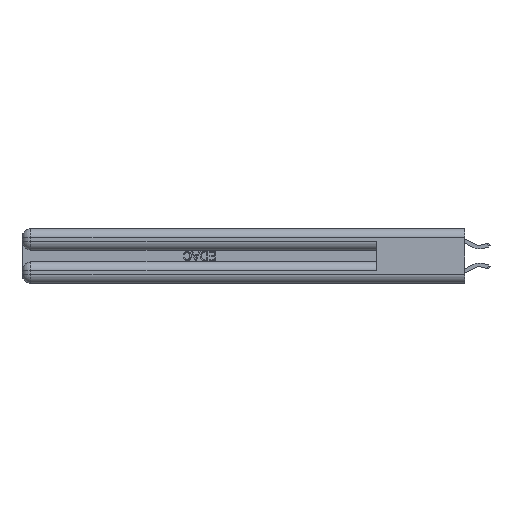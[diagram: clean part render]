
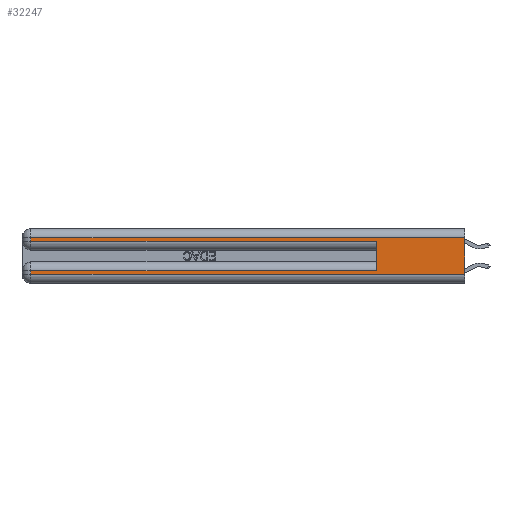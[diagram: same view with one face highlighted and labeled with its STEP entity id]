
A CAD part, left-side view. The second image highlights one B-rep face of the part: STEP entity #32247.
In plain terms, the highlighted planar face has unit normal (-1, 0, 0).
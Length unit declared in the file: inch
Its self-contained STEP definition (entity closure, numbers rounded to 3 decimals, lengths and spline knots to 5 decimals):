
#521 = VERTEX_POINT ( 'NONE', #4528 ) ;
#645 = CARTESIAN_POINT ( 'NONE',  ( 0., 0.6, 0.085 ) ) ;
#839 = CARTESIAN_POINT ( 'NONE',  ( 0., 0., 0.285 ) ) ;
#1564 = DIRECTION ( 'NONE',  ( 0., -1., 0. ) ) ;
#1755 = LINE ( 'NONE', #20086, #27776 ) ;
#1814 = AXIS2_PLACEMENT_3D ( 'NONE', #4807, #31588, #29104 ) ;
#2146 = CARTESIAN_POINT ( 'NONE',  ( 0., 2.94, 0.37 ) ) ;
#2331 = LINE ( 'NONE', #15736, #18131 ) ;
#2772 = LINE ( 'NONE', #21984, #14631 ) ;
#3386 = ORIENTED_EDGE ( 'NONE', *, *, #16109, .T. ) ;
#3832 = CARTESIAN_POINT ( 'NONE',  ( 0., 0., 0.31 ) ) ;
#3846 = VERTEX_POINT ( 'NONE', #17870 ) ;
#4039 = ORIENTED_EDGE ( 'NONE', *, *, #29134, .F. ) ;
#4528 = CARTESIAN_POINT ( 'NONE',  ( 0., 2.94, 0.06 ) ) ;
#4693 = EDGE_CURVE ( 'NONE', #20149, #20709, #12934, .T. ) ;
#4807 = CARTESIAN_POINT ( 'NONE',  ( 0., 0., 0.37 ) ) ;
#5538 = EDGE_CURVE ( 'NONE', #20709, #32707, #14271, .T. ) ;
#5596 = EDGE_CURVE ( 'NONE', #21968, #20149, #15321, .T. ) ;
#6369 = VECTOR ( 'NONE', #26561, 39.37008 ) ;
#7666 = ORIENTED_EDGE ( 'NONE', *, *, #15448, .F. ) ;
#8062 = CARTESIAN_POINT ( 'NONE',  ( 0., 0., 0.31 ) ) ;
#9660 = EDGE_LOOP ( 'NONE', ( #7666, #19116, #23951, #28795, #4039, #12200, #33163, #3386 ) ) ;
#11644 = DIRECTION ( 'NONE',  ( 0., -1., 0. ) ) ;
#12200 = ORIENTED_EDGE ( 'NONE', *, *, #12401, .T. ) ;
#12401 = EDGE_CURVE ( 'NONE', #13423, #26680, #2331, .T. ) ;
#12593 = CARTESIAN_POINT ( 'NONE',  ( 0., 2.94, 0.085 ) ) ;
#12934 = LINE ( 'NONE', #2146, #33450 ) ;
#13423 = VERTEX_POINT ( 'NONE', #645 ) ;
#13480 = LINE ( 'NONE', #21568, #13785 ) ;
#13690 = EDGE_CURVE ( 'NONE', #26680, #521, #31986, .T. ) ;
#13785 = VECTOR ( 'NONE', #31953, 39.37008 ) ;
#14271 = LINE ( 'NONE', #839, #33241 ) ;
#14631 = VECTOR ( 'NONE', #30089, 39.37008 ) ;
#15321 = LINE ( 'NONE', #3832, #25917 ) ;
#15400 = PLANE ( 'NONE',  #1814 ) ;
#15448 = EDGE_CURVE ( 'NONE', #21968, #3846, #13480, .T. ) ;
#15736 = CARTESIAN_POINT ( 'NONE',  ( 0., 0., 0.085 ) ) ;
#15806 = CARTESIAN_POINT ( 'NONE',  ( 0., 2.94, 0.37 ) ) ;
#16109 = EDGE_CURVE ( 'NONE', #521, #3846, #1755, .T. ) ;
#17154 = CARTESIAN_POINT ( 'NONE',  ( 0., 2.94, 0.31 ) ) ;
#17870 = CARTESIAN_POINT ( 'NONE',  ( 0., 0., 0.06 ) ) ;
#18131 = VECTOR ( 'NONE', #26308, 39.37008 ) ;
#19116 = ORIENTED_EDGE ( 'NONE', *, *, #5596, .T. ) ;
#20086 = CARTESIAN_POINT ( 'NONE',  ( 0., 0., 0.06 ) ) ;
#20149 = VERTEX_POINT ( 'NONE', #17154 ) ;
#20709 = VERTEX_POINT ( 'NONE', #34025 ) ;
#21568 = CARTESIAN_POINT ( 'NONE',  ( 0., 0., 0.37 ) ) ;
#21968 = VERTEX_POINT ( 'NONE', #8062 ) ;
#21984 = CARTESIAN_POINT ( 'NONE',  ( 0., 0.6, 0.145 ) ) ;
#23951 = ORIENTED_EDGE ( 'NONE', *, *, #4693, .T. ) ;
#25917 = VECTOR ( 'NONE', #28339, 39.37008 ) ;
#26308 = DIRECTION ( 'NONE',  ( 0., 1., 0. ) ) ;
#26561 = DIRECTION ( 'NONE',  ( 0., 0., -1. ) ) ;
#26680 = VERTEX_POINT ( 'NONE', #12593 ) ;
#27776 = VECTOR ( 'NONE', #1564, 39.37008 ) ;
#28339 = DIRECTION ( 'NONE',  ( 0., 1., 0. ) ) ;
#28795 = ORIENTED_EDGE ( 'NONE', *, *, #5538, .T. ) ;
#29104 = DIRECTION ( 'NONE',  ( 0., 0., -1. ) ) ;
#29134 = EDGE_CURVE ( 'NONE', #13423, #32707, #2772, .T. ) ;
#29243 = CARTESIAN_POINT ( 'NONE',  ( 0., 0.6, 0.285 ) ) ;
#30089 = DIRECTION ( 'NONE',  ( 0., 0., 1. ) ) ;
#31080 = DIRECTION ( 'NONE',  ( 0., 0., -1. ) ) ;
#31588 = DIRECTION ( 'NONE',  ( 1., 0., 0. ) ) ;
#31953 = DIRECTION ( 'NONE',  ( 0., 0., -1. ) ) ;
#31986 = LINE ( 'NONE', #15806, #6369 ) ;
#32247 = ADVANCED_FACE ( 'NONE', ( #34232 ), #15400, .F. ) ;
#32707 = VERTEX_POINT ( 'NONE', #29243 ) ;
#33163 = ORIENTED_EDGE ( 'NONE', *, *, #13690, .T. ) ;
#33241 = VECTOR ( 'NONE', #11644, 39.37008 ) ;
#33450 = VECTOR ( 'NONE', #31080, 39.37008 ) ;
#34025 = CARTESIAN_POINT ( 'NONE',  ( 0., 2.94, 0.285 ) ) ;
#34232 = FACE_OUTER_BOUND ( 'NONE', #9660, .T. ) ;
